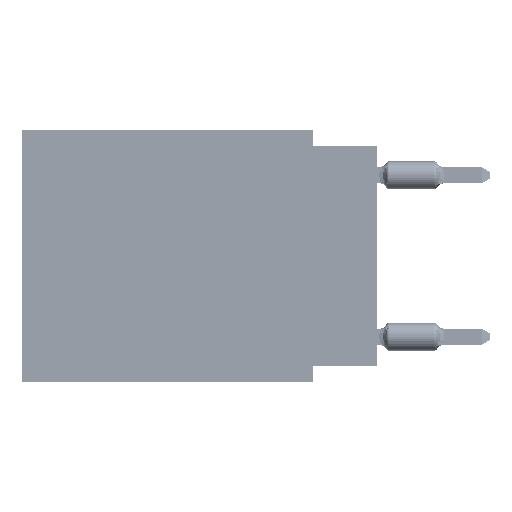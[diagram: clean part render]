
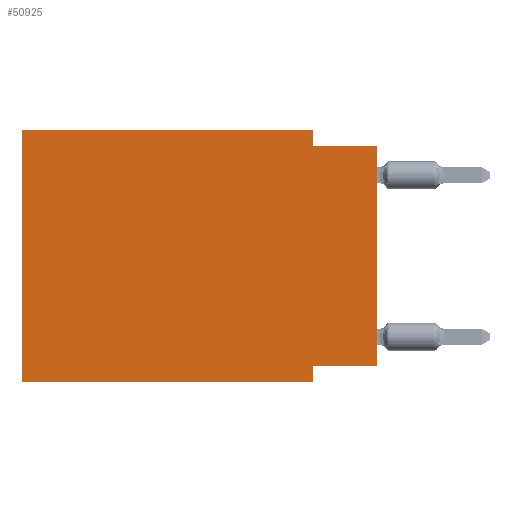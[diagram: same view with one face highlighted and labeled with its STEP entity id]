
A CAD part, left-side view. The second image highlights one B-rep face of the part: STEP entity #50925.
In plain terms, the highlighted planar face has unit normal (-1, 0, 0).
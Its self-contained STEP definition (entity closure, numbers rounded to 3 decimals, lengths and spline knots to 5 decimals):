
#1300 = CARTESIAN_POINT ( 'NONE',  ( 0., 0., 0. ) ) ;
#1932 = CARTESIAN_POINT ( 'NONE',  ( 0., 0.1, -0.39 ) ) ;
#2100 = LINE ( 'NONE', #61730, #53906 ) ;
#4876 = CARTESIAN_POINT ( 'NONE',  ( 0., 0., -0.365 ) ) ;
#6797 = DIRECTION ( 'NONE',  ( 0., 0., -1. ) ) ;
#7336 = DIRECTION ( 'NONE',  ( 0., 0., -1. ) ) ;
#7715 = ORIENTED_EDGE ( 'NONE', *, *, #34932, .F. ) ;
#8060 = LINE ( 'NONE', #1300, #14375 ) ;
#11598 = VECTOR ( 'NONE', #69341, 39.37008 ) ;
#12083 = ORIENTED_EDGE ( 'NONE', *, *, #80997, .F. ) ;
#13889 = VECTOR ( 'NONE', #7336, 39.37008 ) ;
#14375 = VECTOR ( 'NONE', #35398, 39.37008 ) ;
#14554 = LINE ( 'NONE', #20848, #88558 ) ;
#15790 = VECTOR ( 'NONE', #61159, 39.37008 ) ;
#17696 = VECTOR ( 'NONE', #42208, 39.37008 ) ;
#19783 = FACE_OUTER_BOUND ( 'NONE', #43035, .T. ) ;
#19907 = LINE ( 'NONE', #20813, #31695 ) ;
#20813 = CARTESIAN_POINT ( 'NONE',  ( 0., 0.1, 0. ) ) ;
#20848 = CARTESIAN_POINT ( 'NONE',  ( 0., 0., -0.365 ) ) ;
#21545 = CARTESIAN_POINT ( 'NONE',  ( 0., 0.55, 0. ) ) ;
#27286 = CARTESIAN_POINT ( 'NONE',  ( 0., 0.1, -0.39 ) ) ;
#29271 = LINE ( 'NONE', #1932, #13889 ) ;
#30341 = ORIENTED_EDGE ( 'NONE', *, *, #39391, .T. ) ;
#30505 = LINE ( 'NONE', #21545, #17696 ) ;
#30572 = AXIS2_PLACEMENT_3D ( 'NONE', #74543, #68655, #6797 ) ;
#31695 = VECTOR ( 'NONE', #75561, 39.37008 ) ;
#33720 = PLANE ( 'NONE',  #30572 ) ;
#34932 = EDGE_CURVE ( 'NONE', #78692, #86604, #14554, .T. ) ;
#35152 = CARTESIAN_POINT ( 'NONE',  ( 0., 0.55, 0. ) ) ;
#35398 = DIRECTION ( 'NONE',  ( 0., 0., 1. ) ) ;
#39391 = EDGE_CURVE ( 'NONE', #78692, #60562, #8060, .T. ) ;
#40561 = LINE ( 'NONE', #35152, #15790 ) ;
#41131 = CARTESIAN_POINT ( 'NONE',  ( 0., 0.55, -0.39 ) ) ;
#42208 = DIRECTION ( 'NONE',  ( 0., -1., 0. ) ) ;
#43035 = EDGE_LOOP ( 'NONE', ( #30341, #68400, #72082, #84434, #12083, #61429, #84522, #7715 ) ) ;
#44518 = CARTESIAN_POINT ( 'NONE',  ( 0., 0.55, -0.39 ) ) ;
#45149 = VERTEX_POINT ( 'NONE', #27286 ) ;
#47432 = VERTEX_POINT ( 'NONE', #44518 ) ;
#48881 = VERTEX_POINT ( 'NONE', #68091 ) ;
#50138 = CARTESIAN_POINT ( 'NONE',  ( 0., 0.1, -0.025 ) ) ;
#50925 = ADVANCED_FACE ( 'NONE', ( #19783 ), #33720, .F. ) ;
#51115 = EDGE_CURVE ( 'NONE', #52675, #48881, #30505, .T. ) ;
#52675 = VERTEX_POINT ( 'NONE', #66881 ) ;
#53906 = VECTOR ( 'NONE', #70716, 39.37008 ) ;
#55804 = DIRECTION ( 'NONE',  ( 0., 1., 0. ) ) ;
#60562 = VERTEX_POINT ( 'NONE', #85641 ) ;
#61159 = DIRECTION ( 'NONE',  ( 0., 0., 1. ) ) ;
#61429 = ORIENTED_EDGE ( 'NONE', *, *, #86395, .T. ) ;
#61730 = CARTESIAN_POINT ( 'NONE',  ( 0., 0., -0.025 ) ) ;
#65856 = EDGE_CURVE ( 'NONE', #86604, #45149, #29271, .T. ) ;
#66881 = CARTESIAN_POINT ( 'NONE',  ( 0., 0.55, 0. ) ) ;
#68091 = CARTESIAN_POINT ( 'NONE',  ( 0., 0.1, 0. ) ) ;
#68400 = ORIENTED_EDGE ( 'NONE', *, *, #75976, .F. ) ;
#68655 = DIRECTION ( 'NONE',  ( 1., 0., 0. ) ) ;
#69341 = DIRECTION ( 'NONE',  ( 0., -1., 0. ) ) ;
#70716 = DIRECTION ( 'NONE',  ( 0., -1., 0. ) ) ;
#72082 = ORIENTED_EDGE ( 'NONE', *, *, #86864, .F. ) ;
#74543 = CARTESIAN_POINT ( 'NONE',  ( 0., 0.55, 0. ) ) ;
#75561 = DIRECTION ( 'NONE',  ( 0., 0., -1. ) ) ;
#75976 = EDGE_CURVE ( 'NONE', #80811, #60562, #2100, .T. ) ;
#78692 = VERTEX_POINT ( 'NONE', #4876 ) ;
#79632 = CARTESIAN_POINT ( 'NONE',  ( 0., 0.1, -0.365 ) ) ;
#80811 = VERTEX_POINT ( 'NONE', #50138 ) ;
#80997 = EDGE_CURVE ( 'NONE', #47432, #52675, #40561, .T. ) ;
#82399 = LINE ( 'NONE', #41131, #11598 ) ;
#84434 = ORIENTED_EDGE ( 'NONE', *, *, #51115, .F. ) ;
#84522 = ORIENTED_EDGE ( 'NONE', *, *, #65856, .F. ) ;
#85641 = CARTESIAN_POINT ( 'NONE',  ( 0., 0., -0.025 ) ) ;
#86395 = EDGE_CURVE ( 'NONE', #47432, #45149, #82399, .T. ) ;
#86604 = VERTEX_POINT ( 'NONE', #79632 ) ;
#86864 = EDGE_CURVE ( 'NONE', #48881, #80811, #19907, .T. ) ;
#88558 = VECTOR ( 'NONE', #55804, 39.37008 ) ;
